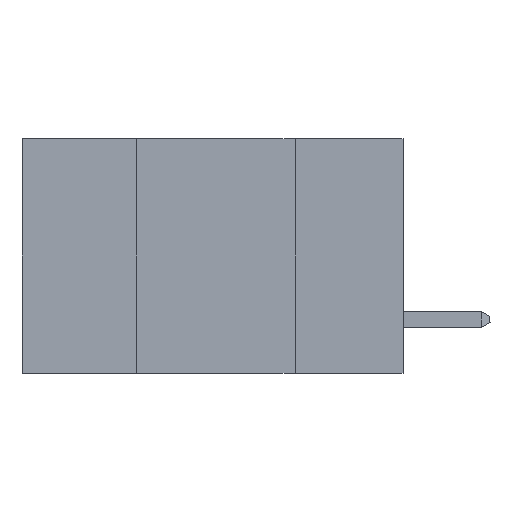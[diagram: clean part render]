
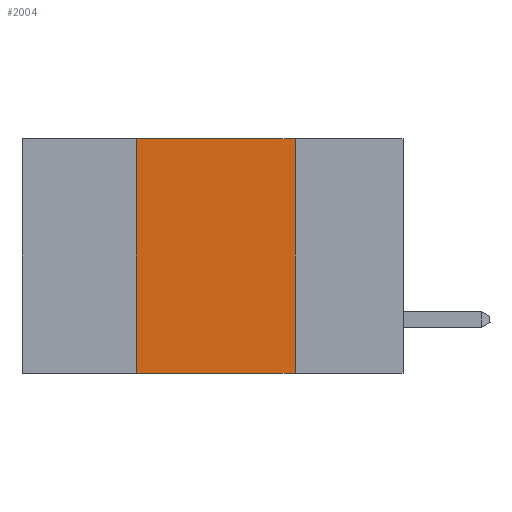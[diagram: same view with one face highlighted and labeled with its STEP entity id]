
A CAD part, left-side view. The second image highlights one B-rep face of the part: STEP entity #2004.
In plain terms, the highlighted planar face has unit normal (-1, 0, 0).
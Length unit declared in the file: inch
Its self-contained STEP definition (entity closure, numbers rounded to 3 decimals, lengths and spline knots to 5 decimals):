
#693 = CARTESIAN_POINT ( 'NONE',  ( 0., 0.17, 0. ) ) ;
#889 = ORIENTED_EDGE ( 'NONE', *, *, #12091, .T. ) ;
#1770 = PLANE ( 'NONE',  #6175 ) ;
#2004 = ADVANCED_FACE ( 'NONE', ( #2746 ), #1770, .F. ) ;
#2132 = LINE ( 'NONE', #8249, #3550 ) ;
#2535 = DIRECTION ( 'NONE',  ( 0., 0., 1. ) ) ;
#2663 = DIRECTION ( 'NONE',  ( 1., 0., 0. ) ) ;
#2746 = FACE_OUTER_BOUND ( 'NONE', #4063, .T. ) ;
#3199 = LINE ( 'NONE', #693, #7658 ) ;
#3266 = DIRECTION ( 'NONE',  ( 0., 0., -1. ) ) ;
#3550 = VECTOR ( 'NONE', #9287, 39.37008 ) ;
#4030 = VERTEX_POINT ( 'NONE', #6069 ) ;
#4063 = EDGE_LOOP ( 'NONE', ( #5939, #11705, #5653, #889 ) ) ;
#5277 = VERTEX_POINT ( 'NONE', #9164 ) ;
#5653 = ORIENTED_EDGE ( 'NONE', *, *, #7338, .F. ) ;
#5848 = EDGE_CURVE ( 'NONE', #5277, #8187, #2132, .T. ) ;
#5939 = ORIENTED_EDGE ( 'NONE', *, *, #11614, .F. ) ;
#6026 = LINE ( 'NONE', #9810, #13047 ) ;
#6069 = CARTESIAN_POINT ( 'NONE',  ( 0., 0.42, -0.37 ) ) ;
#6175 = AXIS2_PLACEMENT_3D ( 'NONE', #12956, #2663, #6820 ) ;
#6820 = DIRECTION ( 'NONE',  ( 0., 0., -1. ) ) ;
#7338 = EDGE_CURVE ( 'NONE', #4030, #5277, #11935, .T. ) ;
#7658 = VECTOR ( 'NONE', #3266, 39.37008 ) ;
#8187 = VERTEX_POINT ( 'NONE', #9851 ) ;
#8249 = CARTESIAN_POINT ( 'NONE',  ( 0., 0.6, 0. ) ) ;
#8717 = CARTESIAN_POINT ( 'NONE',  ( 0., 0.42, 0. ) ) ;
#8933 = VERTEX_POINT ( 'NONE', #10973 ) ;
#9164 = CARTESIAN_POINT ( 'NONE',  ( 0., 0.42, 0. ) ) ;
#9287 = DIRECTION ( 'NONE',  ( 0., -1., 0. ) ) ;
#9409 = VECTOR ( 'NONE', #2535, 39.37008 ) ;
#9810 = CARTESIAN_POINT ( 'NONE',  ( 0., 0.6, -0.37 ) ) ;
#9851 = CARTESIAN_POINT ( 'NONE',  ( 0., 0.17, 0. ) ) ;
#10867 = DIRECTION ( 'NONE',  ( 0., -1., 0. ) ) ;
#10973 = CARTESIAN_POINT ( 'NONE',  ( 0., 0.17, -0.37 ) ) ;
#11614 = EDGE_CURVE ( 'NONE', #8187, #8933, #3199, .T. ) ;
#11705 = ORIENTED_EDGE ( 'NONE', *, *, #5848, .F. ) ;
#11935 = LINE ( 'NONE', #8717, #9409 ) ;
#12091 = EDGE_CURVE ( 'NONE', #4030, #8933, #6026, .T. ) ;
#12956 = CARTESIAN_POINT ( 'NONE',  ( 0., 0.6, 0. ) ) ;
#13047 = VECTOR ( 'NONE', #10867, 39.37008 ) ;
